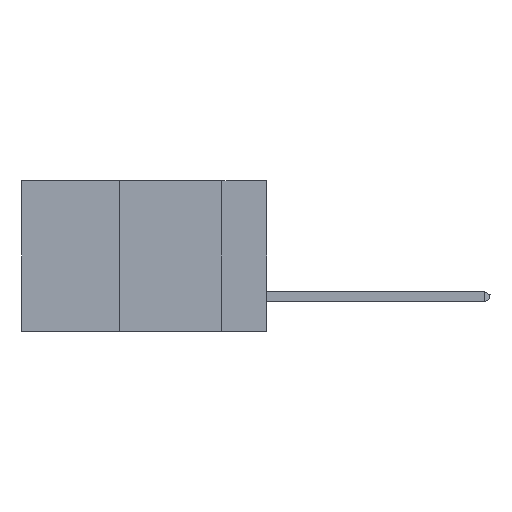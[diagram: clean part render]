
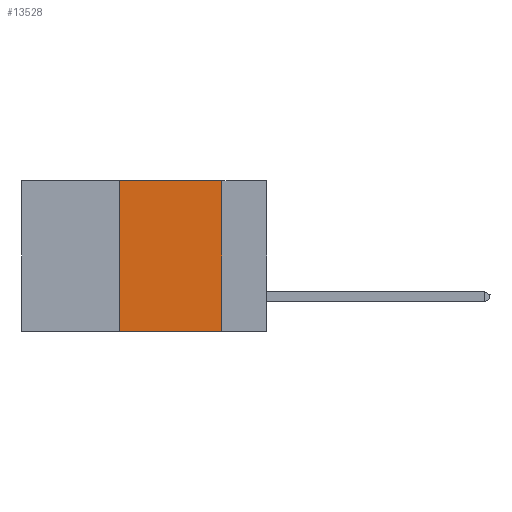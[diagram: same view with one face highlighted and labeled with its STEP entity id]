
A CAD part, left-side view. The second image highlights one B-rep face of the part: STEP entity #13528.
In plain terms, the highlighted planar face has unit normal (-1, 0, 0).
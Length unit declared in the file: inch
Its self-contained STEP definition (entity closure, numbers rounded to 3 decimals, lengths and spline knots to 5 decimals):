
#29 = CARTESIAN_POINT ( 'NONE',  ( 0., 0.36, 0. ) ) ;
#50 = EDGE_CURVE ( 'NONE', #862, #12463, #3976, .T. ) ;
#367 = VECTOR ( 'NONE', #4470, 39.37008 ) ;
#525 = CARTESIAN_POINT ( 'NONE',  ( 0., 0.11, -0.37 ) ) ;
#862 = VERTEX_POINT ( 'NONE', #14260 ) ;
#1120 = EDGE_LOOP ( 'NONE', ( #7557, #1204, #4220, #16049 ) ) ;
#1204 = ORIENTED_EDGE ( 'NONE', *, *, #5782, .F. ) ;
#1254 = DIRECTION ( 'NONE',  ( 0., 0., -1. ) ) ;
#2821 = VERTEX_POINT ( 'NONE', #9321 ) ;
#2999 = CARTESIAN_POINT ( 'NONE',  ( 0., 0.6, 0. ) ) ;
#3976 = LINE ( 'NONE', #17292, #11607 ) ;
#4220 = ORIENTED_EDGE ( 'NONE', *, *, #18375, .F. ) ;
#4470 = DIRECTION ( 'NONE',  ( 0., -1., 0. ) ) ;
#5628 = FACE_OUTER_BOUND ( 'NONE', #1120, .T. ) ;
#5650 = DIRECTION ( 'NONE',  ( 0., -1., 0. ) ) ;
#5782 = EDGE_CURVE ( 'NONE', #11066, #862, #11948, .T. ) ;
#7296 = DIRECTION ( 'NONE',  ( 1., 0., 0. ) ) ;
#7557 = ORIENTED_EDGE ( 'NONE', *, *, #50, .F. ) ;
#8660 = AXIS2_PLACEMENT_3D ( 'NONE', #2999, #7296, #1254 ) ;
#9321 = CARTESIAN_POINT ( 'NONE',  ( 0., 0.36, -0.37 ) ) ;
#9695 = LINE ( 'NONE', #18616, #13279 ) ;
#9827 = DIRECTION ( 'NONE',  ( 0., 0., -1. ) ) ;
#10005 = PLANE ( 'NONE',  #8660 ) ;
#11066 = VERTEX_POINT ( 'NONE', #29 ) ;
#11121 = DIRECTION ( 'NONE',  ( 0., 0., 1. ) ) ;
#11561 = LINE ( 'NONE', #19156, #19059 ) ;
#11607 = VECTOR ( 'NONE', #9827, 39.37008 ) ;
#11948 = LINE ( 'NONE', #16643, #367 ) ;
#12463 = VERTEX_POINT ( 'NONE', #525 ) ;
#13279 = VECTOR ( 'NONE', #11121, 39.37008 ) ;
#13528 = ADVANCED_FACE ( 'NONE', ( #5628 ), #10005, .F. ) ;
#14260 = CARTESIAN_POINT ( 'NONE',  ( 0., 0.11, 0. ) ) ;
#16046 = EDGE_CURVE ( 'NONE', #2821, #12463, #11561, .T. ) ;
#16049 = ORIENTED_EDGE ( 'NONE', *, *, #16046, .T. ) ;
#16643 = CARTESIAN_POINT ( 'NONE',  ( 0., 0.6, 0. ) ) ;
#17292 = CARTESIAN_POINT ( 'NONE',  ( 0., 0.11, 0. ) ) ;
#18375 = EDGE_CURVE ( 'NONE', #2821, #11066, #9695, .T. ) ;
#18616 = CARTESIAN_POINT ( 'NONE',  ( 0., 0.36, 0. ) ) ;
#19059 = VECTOR ( 'NONE', #5650, 39.37008 ) ;
#19156 = CARTESIAN_POINT ( 'NONE',  ( 0., 0.6, -0.37 ) ) ;
